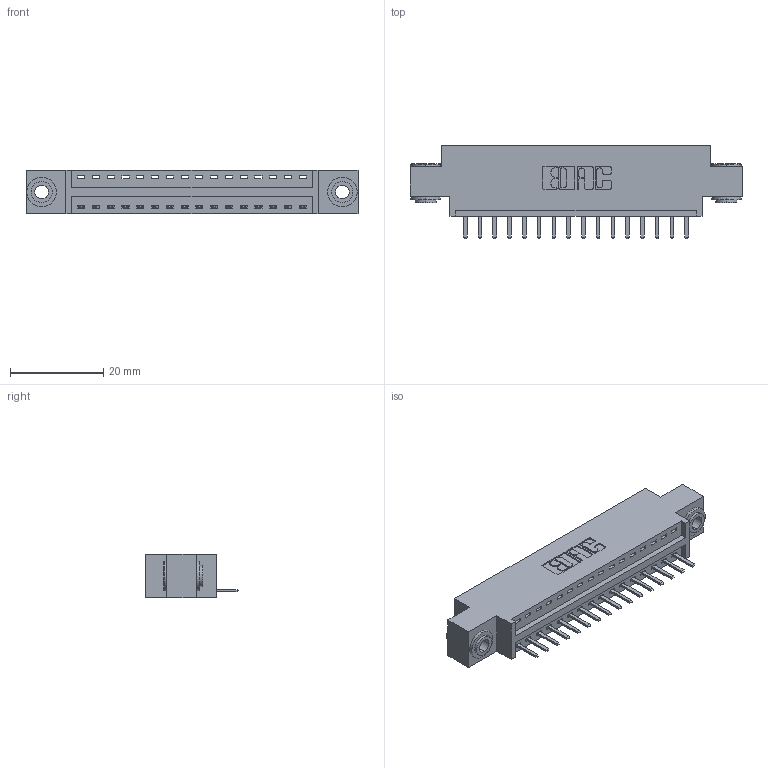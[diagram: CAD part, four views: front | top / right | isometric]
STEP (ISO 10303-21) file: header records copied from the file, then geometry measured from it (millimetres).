
FILE_DESCRIPTION (( 'STEP AP203' ), '1' );
FILE_NAME ('396-016-520-603.STEP', '2019-10-26T17:55:05', ( '' ), ( '' ), 'SwSTEP 2.0', 'SolidWorks 2016', '' );
FILE_SCHEMA (( 'CONFIG_CONTROL_DESIGN' ));
Length unit declared in the file: inch
Products named in the file (4): 346 Part_0.170 Offset - 0.156 Dia-TH; 345-250-002_345-250-002-102; 396-016-520-603; 345-292-001_345-293-120
Assembly tree (19 placements, depth 2):
  396-016-520-603
    346 Part_0.170 Offset - 0.156 Dia-TH
    345-292-001_345-293-120  x16
    345-250-002_345-250-002-102  x2
Bounding box: 71.37 x 20.02 x 9.4 mm (x, y, z)
Volume: 6471.7 mm3; surface area: 8034.1 mm2
Topology: 19 solids, 19 shells, 1156 faces, 3361 edges, 2194 vertices
Faces by surface type: plane 762, cylinder 386, cone 8
Entity records: 14326 total; most frequent: CARTESIAN_POINT 2455, ORIENTED_EDGE 2386, DIRECTION 2215, EDGE_CURVE 1193, LINE 969, VECTOR 969, VERTEX_POINT 790, AXIS2_PLACEMENT_3D 623
